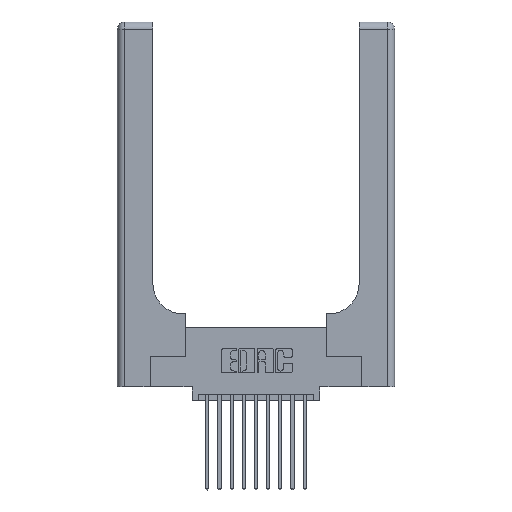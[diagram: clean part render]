
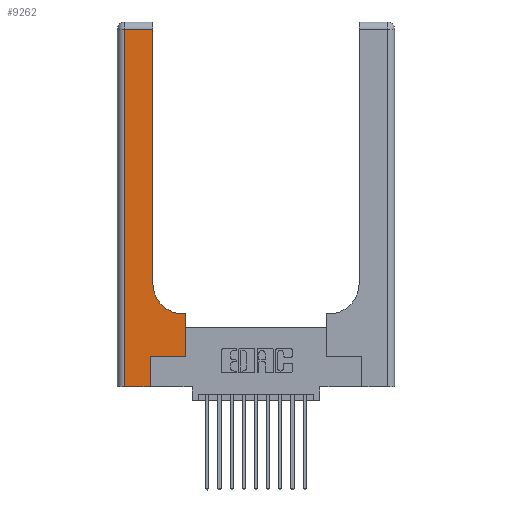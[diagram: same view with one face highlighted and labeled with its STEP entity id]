
A CAD part, top view. The second image highlights one B-rep face of the part: STEP entity #9262.
In plain terms, the highlighted planar face has unit normal (0, 0, 1).
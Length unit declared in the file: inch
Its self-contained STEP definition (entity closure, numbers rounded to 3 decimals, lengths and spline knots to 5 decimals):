
#122 = LINE ( 'NONE', #7028, #7663 ) ;
#450 = CARTESIAN_POINT ( 'NONE',  ( 0.06, 2.94, 0.37 ) ) ;
#782 = DIRECTION ( 'NONE',  ( 0., 1., 0. ) ) ;
#854 = DIRECTION ( 'NONE',  ( 0., -1., 0. ) ) ;
#1078 = ORIENTED_EDGE ( 'NONE', *, *, #7848, .T. ) ;
#1390 = AXIS2_PLACEMENT_3D ( 'NONE', #10718, #12139, #6048 ) ;
#1509 = CARTESIAN_POINT ( 'NONE',  ( 0.269, 0.25, 0.37 ) ) ;
#1837 = LINE ( 'NONE', #9819, #4275 ) ;
#1963 = VECTOR ( 'NONE', #782, 39.37008 ) ;
#2193 = CARTESIAN_POINT ( 'NONE',  ( 0., 0., 0.37 ) ) ;
#2251 = DIRECTION ( 'NONE',  ( 1., 0., 0. ) ) ;
#2299 = VERTEX_POINT ( 'NONE', #12369 ) ;
#2465 = CARTESIAN_POINT ( 'NONE',  ( 0.269, 0.25, 0.37 ) ) ;
#2487 = EDGE_CURVE ( 'NONE', #11355, #2299, #13888, .T. ) ;
#2602 = VECTOR ( 'NONE', #854, 39.37008 ) ;
#2720 = VERTEX_POINT ( 'NONE', #450 ) ;
#2811 = ORIENTED_EDGE ( 'NONE', *, *, #12022, .T. ) ;
#2844 = AXIS2_PLACEMENT_3D ( 'NONE', #6727, #5258, #14329 ) ;
#2930 = CARTESIAN_POINT ( 'NONE',  ( 0.5415, 0.6, 0.37 ) ) ;
#3766 = LINE ( 'NONE', #7430, #13519 ) ;
#3802 = VECTOR ( 'NONE', #7557, 39.37008 ) ;
#3850 = VECTOR ( 'NONE', #2251, 39.37008 ) ;
#3879 = PLANE ( 'NONE',  #1390 ) ;
#3908 = VECTOR ( 'NONE', #14693, 39.37008 ) ;
#3978 = VERTEX_POINT ( 'NONE', #14503 ) ;
#4275 = VECTOR ( 'NONE', #8570, 39.37008 ) ;
#4481 = DIRECTION ( 'NONE',  ( 0., 1., 0. ) ) ;
#4698 = EDGE_CURVE ( 'NONE', #9023, #11355, #1837, .T. ) ;
#4943 = CARTESIAN_POINT ( 'NONE',  ( 0., 2.94, 0.37 ) ) ;
#5063 = EDGE_CURVE ( 'NONE', #13570, #9023, #5095, .T. ) ;
#5095 = LINE ( 'NONE', #2193, #3850 ) ;
#5258 = DIRECTION ( 'NONE',  ( 0., 0., -1. ) ) ;
#6048 = DIRECTION ( 'NONE',  ( -1., 0., 0. ) ) ;
#6182 = DIRECTION ( 'NONE',  ( -1., 0., 0. ) ) ;
#6217 = ORIENTED_EDGE ( 'NONE', *, *, #4698, .T. ) ;
#6667 = ORIENTED_EDGE ( 'NONE', *, *, #7244, .T. ) ;
#6727 = CARTESIAN_POINT ( 'NONE',  ( 0.5415, 0.85, 0.37 ) ) ;
#7028 = CARTESIAN_POINT ( 'NONE',  ( 0.2915, 3., 0.37 ) ) ;
#7244 = EDGE_CURVE ( 'NONE', #2720, #13570, #14796, .T. ) ;
#7255 = CARTESIAN_POINT ( 'NONE',  ( 0.5585, 0.25, 0.37 ) ) ;
#7402 = ORIENTED_EDGE ( 'NONE', *, *, #5063, .T. ) ;
#7430 = CARTESIAN_POINT ( 'NONE',  ( 0.2915, 0.6, 0.37 ) ) ;
#7557 = DIRECTION ( 'NONE',  ( -1., 0., 0. ) ) ;
#7663 = VECTOR ( 'NONE', #4481, 39.37008 ) ;
#7848 = EDGE_CURVE ( 'NONE', #16471, #2720, #12969, .T. ) ;
#7856 = CARTESIAN_POINT ( 'NONE',  ( 0.5585, 0.6, 0.37 ) ) ;
#7901 = EDGE_LOOP ( 'NONE', ( #9250, #1078, #6667, #7402, #6217, #8645, #11255, #12579, #2811 ) ) ;
#7939 = VERTEX_POINT ( 'NONE', #2930 ) ;
#8274 = CARTESIAN_POINT ( 'NONE',  ( 0.269, 0., 0.37 ) ) ;
#8560 = EDGE_CURVE ( 'NONE', #3978, #16471, #122, .T. ) ;
#8570 = DIRECTION ( 'NONE',  ( 0., 1., 0. ) ) ;
#8645 = ORIENTED_EDGE ( 'NONE', *, *, #2487, .T. ) ;
#9023 = VERTEX_POINT ( 'NONE', #8274 ) ;
#9250 = ORIENTED_EDGE ( 'NONE', *, *, #8560, .T. ) ;
#9262 = ADVANCED_FACE ( 'NONE', ( #13908 ), #3879, .F. ) ;
#9819 = CARTESIAN_POINT ( 'NONE',  ( 0.269, 0., 0.37 ) ) ;
#10718 = CARTESIAN_POINT ( 'NONE',  ( 0., 3., 0.37 ) ) ;
#11255 = ORIENTED_EDGE ( 'NONE', *, *, #14472, .T. ) ;
#11355 = VERTEX_POINT ( 'NONE', #2465 ) ;
#11484 = VERTEX_POINT ( 'NONE', #7856 ) ;
#12022 = EDGE_CURVE ( 'NONE', #7939, #3978, #15681, .T. ) ;
#12139 = DIRECTION ( 'NONE',  ( 0., 0., -1. ) ) ;
#12339 = LINE ( 'NONE', #7255, #1963 ) ;
#12369 = CARTESIAN_POINT ( 'NONE',  ( 0.5585, 0.25, 0.37 ) ) ;
#12579 = ORIENTED_EDGE ( 'NONE', *, *, #14669, .T. ) ;
#12762 = CARTESIAN_POINT ( 'NONE',  ( 0.06, 0., 0.37 ) ) ;
#12969 = LINE ( 'NONE', #4943, #3802 ) ;
#13519 = VECTOR ( 'NONE', #6182, 39.37008 ) ;
#13570 = VERTEX_POINT ( 'NONE', #12762 ) ;
#13796 = CARTESIAN_POINT ( 'NONE',  ( 0.06, 3., 0.37 ) ) ;
#13888 = LINE ( 'NONE', #1509, #3908 ) ;
#13908 = FACE_OUTER_BOUND ( 'NONE', #7901, .T. ) ;
#14329 = DIRECTION ( 'NONE',  ( 1., 0., 0. ) ) ;
#14472 = EDGE_CURVE ( 'NONE', #2299, #11484, #12339, .T. ) ;
#14503 = CARTESIAN_POINT ( 'NONE',  ( 0.2915, 0.85, 0.37 ) ) ;
#14669 = EDGE_CURVE ( 'NONE', #11484, #7939, #3766, .T. ) ;
#14693 = DIRECTION ( 'NONE',  ( 1., 0., 0. ) ) ;
#14796 = LINE ( 'NONE', #13796, #2602 ) ;
#15681 = CIRCLE ( 'NONE', #2844, 0.25 ) ;
#16356 = CARTESIAN_POINT ( 'NONE',  ( 0.2915, 2.94, 0.37 ) ) ;
#16471 = VERTEX_POINT ( 'NONE', #16356 ) ;
